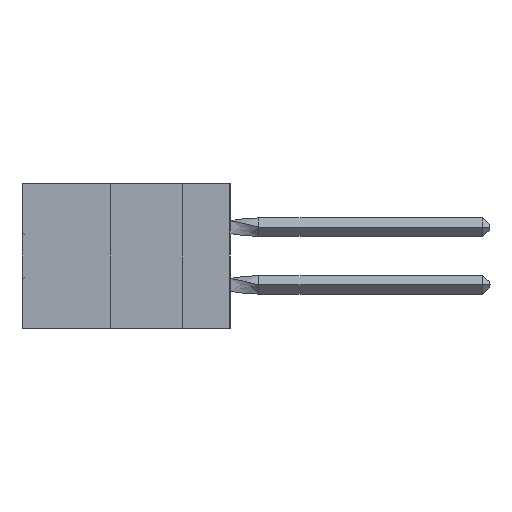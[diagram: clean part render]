
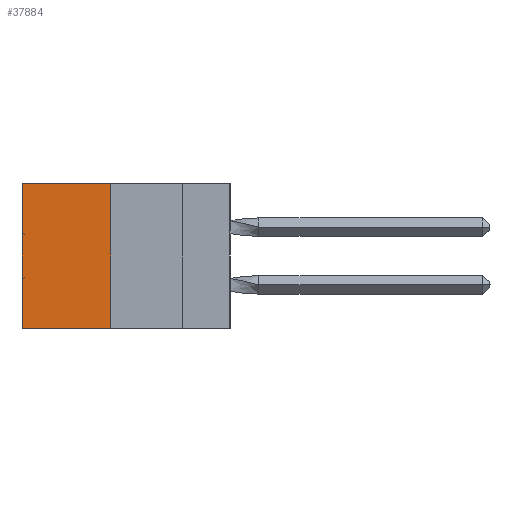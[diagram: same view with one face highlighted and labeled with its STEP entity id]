
A CAD part, left-side view. The second image highlights one B-rep face of the part: STEP entity #37884.
In plain terms, the highlighted planar face has unit normal (-1, 0, 0).
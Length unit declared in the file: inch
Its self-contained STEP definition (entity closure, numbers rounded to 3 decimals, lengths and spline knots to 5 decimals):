
#24 = DIRECTION ( 'NONE',  ( 0., 1., 0. ) ) ;
#504 = EDGE_CURVE ( 'NONE', #20254, #46858, #35012, .T. ) ;
#1032 = EDGE_CURVE ( 'NONE', #20254, #29414, #55182, .T. ) ;
#1992 = ORIENTED_EDGE ( 'NONE', *, *, #1032, .F. ) ;
#2505 = EDGE_LOOP ( 'NONE', ( #32046, #53160, #1992, #36509 ) ) ;
#2649 = VERTEX_POINT ( 'NONE', #17733 ) ;
#5875 = CARTESIAN_POINT ( 'NONE',  ( 0.305, 0.413, -0.5 ) ) ;
#8556 = DIRECTION ( 'NONE',  ( 0., 0., -1. ) ) ;
#8560 = CARTESIAN_POINT ( 'NONE',  ( 0.305, 0.413, 0. ) ) ;
#11377 = DIRECTION ( 'NONE',  ( 0., 0., -1. ) ) ;
#12289 = VECTOR ( 'NONE', #8556, 39.37008 ) ;
#13123 = CARTESIAN_POINT ( 'NONE',  ( 0.305, 0.72, -0.5 ) ) ;
#13450 = LINE ( 'NONE', #44733, #45708 ) ;
#17733 = CARTESIAN_POINT ( 'NONE',  ( 0.305, 0.72, -0.5 ) ) ;
#20025 = LINE ( 'NONE', #13123, #12289 ) ;
#20254 = VERTEX_POINT ( 'NONE', #8560 ) ;
#27451 = AXIS2_PLACEMENT_3D ( 'NONE', #42533, #55757, #11377 ) ;
#29414 = VERTEX_POINT ( 'NONE', #57595 ) ;
#32046 = ORIENTED_EDGE ( 'NONE', *, *, #42584, .T. ) ;
#32747 = CARTESIAN_POINT ( 'NONE',  ( 0.305, 0.72, 0. ) ) ;
#34905 = VECTOR ( 'NONE', #55387, 39.37008 ) ;
#35012 = LINE ( 'NONE', #47141, #54294 ) ;
#36043 = EDGE_CURVE ( 'NONE', #29414, #2649, #13450, .T. ) ;
#36509 = ORIENTED_EDGE ( 'NONE', *, *, #504, .T. ) ;
#37884 = ADVANCED_FACE ( 'NONE', ( #48177 ), #46610, .F. ) ;
#42533 = CARTESIAN_POINT ( 'NONE',  ( 0.305, 0.413, -0.5 ) ) ;
#42584 = EDGE_CURVE ( 'NONE', #46858, #2649, #20025, .T. ) ;
#44733 = CARTESIAN_POINT ( 'NONE',  ( 0.305, 0.413, -0.5 ) ) ;
#45708 = VECTOR ( 'NONE', #24, 39.37008 ) ;
#46610 = PLANE ( 'NONE',  #27451 ) ;
#46858 = VERTEX_POINT ( 'NONE', #32747 ) ;
#47141 = CARTESIAN_POINT ( 'NONE',  ( 0.305, 0.413, 0. ) ) ;
#48177 = FACE_OUTER_BOUND ( 'NONE', #2505, .T. ) ;
#52952 = DIRECTION ( 'NONE',  ( 0., 1., 0. ) ) ;
#53160 = ORIENTED_EDGE ( 'NONE', *, *, #36043, .F. ) ;
#54294 = VECTOR ( 'NONE', #52952, 39.37008 ) ;
#55182 = LINE ( 'NONE', #5875, #34905 ) ;
#55387 = DIRECTION ( 'NONE',  ( 0., 0., -1. ) ) ;
#55757 = DIRECTION ( 'NONE',  ( 1., 0., 0. ) ) ;
#57595 = CARTESIAN_POINT ( 'NONE',  ( 0.305, 0.413, -0.5 ) ) ;
